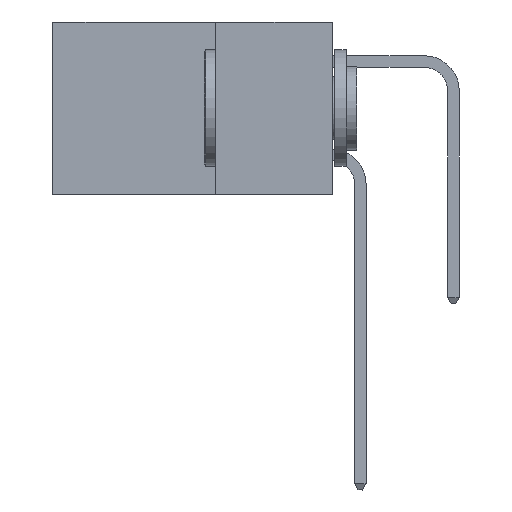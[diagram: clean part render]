
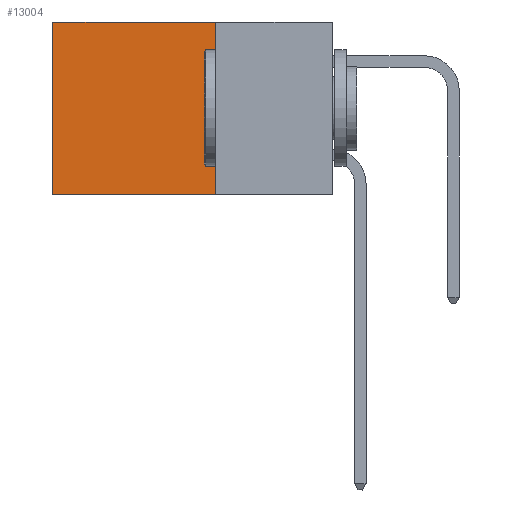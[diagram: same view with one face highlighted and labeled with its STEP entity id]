
A CAD part, left-side view. The second image highlights one B-rep face of the part: STEP entity #13004.
In plain terms, the highlighted planar face has unit normal (-1, 0, 0).
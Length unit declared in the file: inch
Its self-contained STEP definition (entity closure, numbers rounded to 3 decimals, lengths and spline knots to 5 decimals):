
#1611 = VECTOR ( 'NONE', #2783, 39.37008 ) ;
#1693 = DIRECTION ( 'NONE',  ( 0., 0., -1. ) ) ;
#1876 = DIRECTION ( 'NONE',  ( 0., 1., 0. ) ) ;
#2579 = LINE ( 'NONE', #13390, #9161 ) ;
#2692 = VERTEX_POINT ( 'NONE', #6364 ) ;
#2772 = AXIS2_PLACEMENT_3D ( 'NONE', #2988, #10045, #1693 ) ;
#2783 = DIRECTION ( 'NONE',  ( 0., 0., -1. ) ) ;
#2953 = EDGE_LOOP ( 'NONE', ( #16426, #14935, #15099, #5042 ) ) ;
#2988 = CARTESIAN_POINT ( 'NONE',  ( 0.298, 0.25, 0. ) ) ;
#4978 = EDGE_CURVE ( 'NONE', #2692, #13762, #2579, .T. ) ;
#5042 = ORIENTED_EDGE ( 'NONE', *, *, #4978, .T. ) ;
#6039 = EDGE_CURVE ( 'NONE', #13762, #15537, #6659, .T. ) ;
#6364 = CARTESIAN_POINT ( 'NONE',  ( 0.298, 0.25, 0. ) ) ;
#6659 = LINE ( 'NONE', #7188, #13837 ) ;
#6816 = VERTEX_POINT ( 'NONE', #12652 ) ;
#7188 = CARTESIAN_POINT ( 'NONE',  ( 0.298, 0.6, 0. ) ) ;
#7875 = CARTESIAN_POINT ( 'NONE',  ( 0.298, 0.6, -0.37 ) ) ;
#8195 = DIRECTION ( 'NONE',  ( 0., 0., -1. ) ) ;
#8641 = PLANE ( 'NONE',  #2772 ) ;
#8868 = CARTESIAN_POINT ( 'NONE',  ( 0.298, 0.6, 0. ) ) ;
#9161 = VECTOR ( 'NONE', #1876, 39.37008 ) ;
#9561 = VECTOR ( 'NONE', #16844, 39.37008 ) ;
#9769 = CARTESIAN_POINT ( 'NONE',  ( 0.298, 0.25, 0. ) ) ;
#10045 = DIRECTION ( 'NONE',  ( 1., 0., 0. ) ) ;
#10304 = FACE_OUTER_BOUND ( 'NONE', #2953, .T. ) ;
#10361 = EDGE_CURVE ( 'NONE', #6816, #15537, #13890, .T. ) ;
#11601 = CARTESIAN_POINT ( 'NONE',  ( 0.298, 0.25, -0.37 ) ) ;
#12263 = EDGE_CURVE ( 'NONE', #2692, #6816, #16482, .T. ) ;
#12652 = CARTESIAN_POINT ( 'NONE',  ( 0.298, 0.25, -0.37 ) ) ;
#13004 = ADVANCED_FACE ( 'NONE', ( #10304 ), #8641, .F. ) ;
#13390 = CARTESIAN_POINT ( 'NONE',  ( 0.298, 0.25, 0. ) ) ;
#13762 = VERTEX_POINT ( 'NONE', #8868 ) ;
#13837 = VECTOR ( 'NONE', #8195, 39.37008 ) ;
#13890 = LINE ( 'NONE', #11601, #9561 ) ;
#14935 = ORIENTED_EDGE ( 'NONE', *, *, #10361, .F. ) ;
#15099 = ORIENTED_EDGE ( 'NONE', *, *, #12263, .F. ) ;
#15537 = VERTEX_POINT ( 'NONE', #7875 ) ;
#16426 = ORIENTED_EDGE ( 'NONE', *, *, #6039, .T. ) ;
#16482 = LINE ( 'NONE', #9769, #1611 ) ;
#16844 = DIRECTION ( 'NONE',  ( 0., 1., 0. ) ) ;
